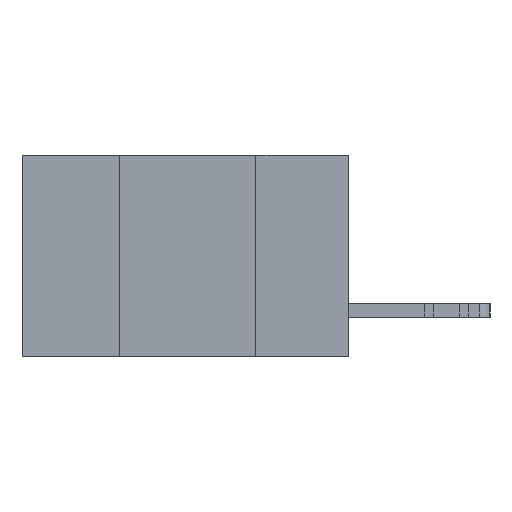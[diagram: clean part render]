
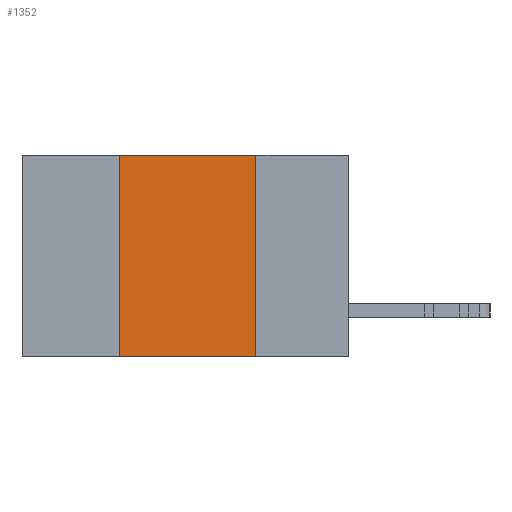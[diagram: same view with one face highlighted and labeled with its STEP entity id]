
A CAD part, left-side view. The second image highlights one B-rep face of the part: STEP entity #1352.
In plain terms, the highlighted planar face has unit normal (-1, 0, 0).
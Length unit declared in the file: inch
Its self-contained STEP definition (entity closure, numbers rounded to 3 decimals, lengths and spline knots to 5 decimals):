
#341 = EDGE_LOOP ( 'NONE', ( #13162, #12916, #3656, #20728 ) ) ;
#1352 = ADVANCED_FACE ( 'NONE', ( #16678 ), #5421, .F. ) ;
#1842 = CARTESIAN_POINT ( 'NONE',  ( 0., 0.17, 0. ) ) ;
#2500 = EDGE_CURVE ( 'NONE', #21438, #11360, #26389, .T. ) ;
#2859 = CARTESIAN_POINT ( 'NONE',  ( 0., 0.17, -0.37 ) ) ;
#3107 = CARTESIAN_POINT ( 'NONE',  ( 0., 0.17, 0. ) ) ;
#3656 = ORIENTED_EDGE ( 'NONE', *, *, #2500, .F. ) ;
#5421 = PLANE ( 'NONE',  #13226 ) ;
#5491 = VERTEX_POINT ( 'NONE', #3107 ) ;
#5611 = DIRECTION ( 'NONE',  ( 0., 0., -1. ) ) ;
#7243 = VECTOR ( 'NONE', #19395, 39.37008 ) ;
#7246 = VECTOR ( 'NONE', #12914, 39.37008 ) ;
#7493 = EDGE_CURVE ( 'NONE', #21438, #15134, #8695, .T. ) ;
#8695 = LINE ( 'NONE', #22095, #16828 ) ;
#10533 = DIRECTION ( 'NONE',  ( 1., 0., 0. ) ) ;
#11360 = VERTEX_POINT ( 'NONE', #19387 ) ;
#12914 = DIRECTION ( 'NONE',  ( 0., 0., -1. ) ) ;
#12916 = ORIENTED_EDGE ( 'NONE', *, *, #27623, .F. ) ;
#13043 = LINE ( 'NONE', #15035, #7243 ) ;
#13162 = ORIENTED_EDGE ( 'NONE', *, *, #19482, .F. ) ;
#13226 = AXIS2_PLACEMENT_3D ( 'NONE', #20991, #10533, #5611 ) ;
#14760 = CARTESIAN_POINT ( 'NONE',  ( 0., 0.42, -0.37 ) ) ;
#14906 = VECTOR ( 'NONE', #27303, 39.37008 ) ;
#15035 = CARTESIAN_POINT ( 'NONE',  ( 0., 0.6, 0. ) ) ;
#15134 = VERTEX_POINT ( 'NONE', #2859 ) ;
#15516 = DIRECTION ( 'NONE',  ( 0., -1., 0. ) ) ;
#16678 = FACE_OUTER_BOUND ( 'NONE', #341, .T. ) ;
#16828 = VECTOR ( 'NONE', #15516, 39.37008 ) ;
#19387 = CARTESIAN_POINT ( 'NONE',  ( 0., 0.42, 0. ) ) ;
#19395 = DIRECTION ( 'NONE',  ( 0., -1., 0. ) ) ;
#19482 = EDGE_CURVE ( 'NONE', #5491, #15134, #24521, .T. ) ;
#20728 = ORIENTED_EDGE ( 'NONE', *, *, #7493, .T. ) ;
#20991 = CARTESIAN_POINT ( 'NONE',  ( 0., 0.6, 0. ) ) ;
#21438 = VERTEX_POINT ( 'NONE', #14760 ) ;
#22095 = CARTESIAN_POINT ( 'NONE',  ( 0., 0.6, -0.37 ) ) ;
#24521 = LINE ( 'NONE', #1842, #7246 ) ;
#26389 = LINE ( 'NONE', #27099, #14906 ) ;
#27099 = CARTESIAN_POINT ( 'NONE',  ( 0., 0.42, 0. ) ) ;
#27303 = DIRECTION ( 'NONE',  ( 0., 0., 1. ) ) ;
#27623 = EDGE_CURVE ( 'NONE', #11360, #5491, #13043, .T. ) ;
